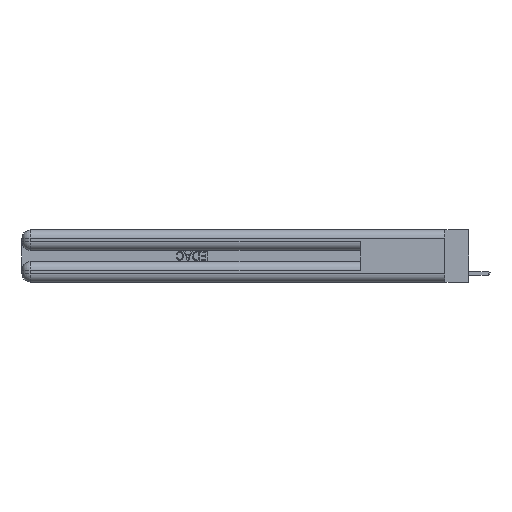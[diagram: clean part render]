
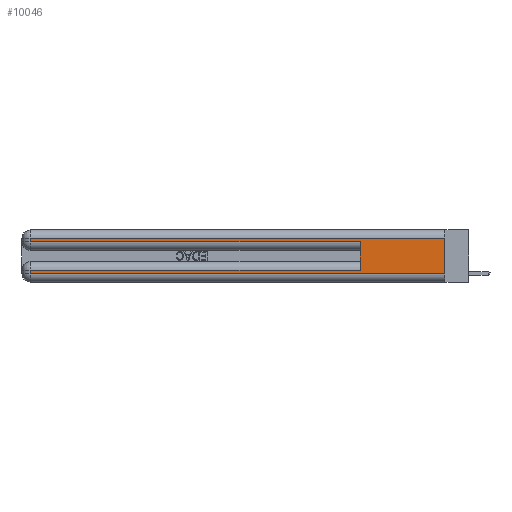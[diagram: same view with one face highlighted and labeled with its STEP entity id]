
A CAD part, left-side view. The second image highlights one B-rep face of the part: STEP entity #10046.
In plain terms, the highlighted planar face has unit normal (-1, 0, 0).
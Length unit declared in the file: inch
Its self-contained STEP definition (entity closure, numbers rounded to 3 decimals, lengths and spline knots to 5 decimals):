
#221 = EDGE_CURVE ( 'NONE', #20258, #16551, #14357, .T. ) ;
#355 = VECTOR ( 'NONE', #21431, 39.37008 ) ;
#777 = DIRECTION ( 'NONE',  ( 1., 0., 0. ) ) ;
#2457 = VECTOR ( 'NONE', #23533, 39.37008 ) ;
#2491 = DIRECTION ( 'NONE',  ( 0., 1., 0. ) ) ;
#3009 = ORIENTED_EDGE ( 'NONE', *, *, #3302, .T. ) ;
#3037 = EDGE_CURVE ( 'NONE', #17451, #26753, #28538, .T. ) ;
#3050 = LINE ( 'NONE', #10661, #25444 ) ;
#3302 = EDGE_CURVE ( 'NONE', #31637, #17451, #27450, .T. ) ;
#3405 = DIRECTION ( 'NONE',  ( 0., 0., -1. ) ) ;
#3719 = ORIENTED_EDGE ( 'NONE', *, *, #24704, .T. ) ;
#3762 = CARTESIAN_POINT ( 'NONE',  ( 0., 2.94, 0.06 ) ) ;
#4163 = CARTESIAN_POINT ( 'NONE',  ( 0., 0., 0.285 ) ) ;
#4237 = VECTOR ( 'NONE', #3405, 39.37008 ) ;
#4623 = VECTOR ( 'NONE', #23689, 39.37008 ) ;
#4818 = ORIENTED_EDGE ( 'NONE', *, *, #5585, .T. ) ;
#4963 = LINE ( 'NONE', #9678, #355 ) ;
#5585 = EDGE_CURVE ( 'NONE', #26753, #29051, #34880, .T. ) ;
#6372 = CARTESIAN_POINT ( 'NONE',  ( 0., 2.94, 0.37 ) ) ;
#8607 = ORIENTED_EDGE ( 'NONE', *, *, #221, .T. ) ;
#8759 = CARTESIAN_POINT ( 'NONE',  ( 0., 0.6, 0.285 ) ) ;
#9137 = ORIENTED_EDGE ( 'NONE', *, *, #26696, .T. ) ;
#9582 = LINE ( 'NONE', #31607, #4623 ) ;
#9678 = CARTESIAN_POINT ( 'NONE',  ( 0., 0.6, 0.145 ) ) ;
#10046 = ADVANCED_FACE ( 'NONE', ( #22685 ), #14897, .F. ) ;
#10661 = CARTESIAN_POINT ( 'NONE',  ( 0., 0., 0.085 ) ) ;
#10860 = EDGE_CURVE ( 'NONE', #30589, #29051, #4963, .T. ) ;
#10950 = CARTESIAN_POINT ( 'NONE',  ( 0., 0., 0.31 ) ) ;
#12575 = LINE ( 'NONE', #31182, #32970 ) ;
#14276 = VECTOR ( 'NONE', #14537, 39.37008 ) ;
#14357 = LINE ( 'NONE', #6372, #14276 ) ;
#14537 = DIRECTION ( 'NONE',  ( 0., 0., -1. ) ) ;
#14544 = CARTESIAN_POINT ( 'NONE',  ( 0., 0., 0.37 ) ) ;
#14897 = PLANE ( 'NONE',  #18310 ) ;
#15017 = VERTEX_POINT ( 'NONE', #29635 ) ;
#16551 = VERTEX_POINT ( 'NONE', #3762 ) ;
#17046 = EDGE_CURVE ( 'NONE', #31637, #15017, #12575, .T. ) ;
#17451 = VERTEX_POINT ( 'NONE', #22492 ) ;
#17790 = EDGE_LOOP ( 'NONE', ( #21151, #3009, #24625, #4818, #33635, #9137, #8607, #3719 ) ) ;
#18310 = AXIS2_PLACEMENT_3D ( 'NONE', #14544, #777, #31132 ) ;
#19902 = CARTESIAN_POINT ( 'NONE',  ( 0., 2.94, 0.37 ) ) ;
#20193 = DIRECTION ( 'NONE',  ( 0., 0., -1. ) ) ;
#20258 = VERTEX_POINT ( 'NONE', #21611 ) ;
#21151 = ORIENTED_EDGE ( 'NONE', *, *, #17046, .F. ) ;
#21431 = DIRECTION ( 'NONE',  ( 0., 0., 1. ) ) ;
#21611 = CARTESIAN_POINT ( 'NONE',  ( 0., 2.94, 0.085 ) ) ;
#22024 = CARTESIAN_POINT ( 'NONE',  ( 0., 0., 0.31 ) ) ;
#22492 = CARTESIAN_POINT ( 'NONE',  ( 0., 2.94, 0.31 ) ) ;
#22685 = FACE_OUTER_BOUND ( 'NONE', #17790, .T. ) ;
#23533 = DIRECTION ( 'NONE',  ( 0., -1., 0. ) ) ;
#23689 = DIRECTION ( 'NONE',  ( 0., -1., 0. ) ) ;
#24595 = CARTESIAN_POINT ( 'NONE',  ( 0., 2.94, 0.285 ) ) ;
#24625 = ORIENTED_EDGE ( 'NONE', *, *, #3037, .T. ) ;
#24704 = EDGE_CURVE ( 'NONE', #16551, #15017, #9582, .T. ) ;
#25444 = VECTOR ( 'NONE', #35406, 39.37008 ) ;
#26620 = CARTESIAN_POINT ( 'NONE',  ( 0., 0.6, 0.085 ) ) ;
#26696 = EDGE_CURVE ( 'NONE', #30589, #20258, #3050, .T. ) ;
#26753 = VERTEX_POINT ( 'NONE', #24595 ) ;
#27450 = LINE ( 'NONE', #22024, #30378 ) ;
#28538 = LINE ( 'NONE', #19902, #4237 ) ;
#29051 = VERTEX_POINT ( 'NONE', #8759 ) ;
#29635 = CARTESIAN_POINT ( 'NONE',  ( 0., 0., 0.06 ) ) ;
#30378 = VECTOR ( 'NONE', #2491, 39.37008 ) ;
#30589 = VERTEX_POINT ( 'NONE', #26620 ) ;
#31132 = DIRECTION ( 'NONE',  ( 0., 0., -1. ) ) ;
#31182 = CARTESIAN_POINT ( 'NONE',  ( 0., 0., 0.37 ) ) ;
#31607 = CARTESIAN_POINT ( 'NONE',  ( 0., 0., 0.06 ) ) ;
#31637 = VERTEX_POINT ( 'NONE', #10950 ) ;
#32970 = VECTOR ( 'NONE', #20193, 39.37008 ) ;
#33635 = ORIENTED_EDGE ( 'NONE', *, *, #10860, .F. ) ;
#34880 = LINE ( 'NONE', #4163, #2457 ) ;
#35406 = DIRECTION ( 'NONE',  ( 0., 1., 0. ) ) ;
